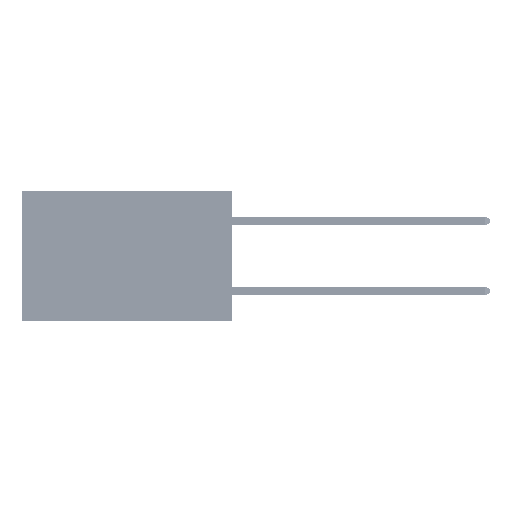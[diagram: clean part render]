
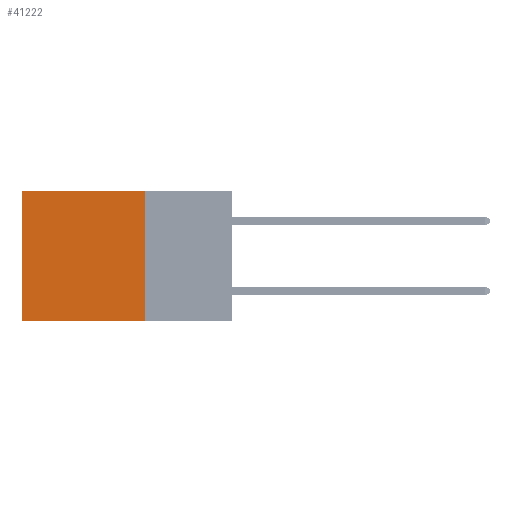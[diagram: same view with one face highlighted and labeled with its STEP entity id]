
A CAD part, left-side view. The second image highlights one B-rep face of the part: STEP entity #41222.
In plain terms, the highlighted planar face has unit normal (-1, 0, 0).
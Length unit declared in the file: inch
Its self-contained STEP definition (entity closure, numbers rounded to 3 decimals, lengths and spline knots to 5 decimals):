
#3738 = DIRECTION ( 'NONE',  ( 0., 1., 0. ) ) ;
#4277 = AXIS2_PLACEMENT_3D ( 'NONE', #21222, #21552, #17971 ) ;
#8140 = VERTEX_POINT ( 'NONE', #16720 ) ;
#9993 = ORIENTED_EDGE ( 'NONE', *, *, #18196, .F. ) ;
#10062 = ORIENTED_EDGE ( 'NONE', *, *, #41769, .T. ) ;
#10303 = LINE ( 'NONE', #29933, #22458 ) ;
#11612 = CARTESIAN_POINT ( 'NONE',  ( 0.2875, 0.6, -0.37 ) ) ;
#13410 = CARTESIAN_POINT ( 'NONE',  ( 0.2875, 0.25, 0. ) ) ;
#13441 = VECTOR ( 'NONE', #30210, 39.37008 ) ;
#13952 = FACE_OUTER_BOUND ( 'NONE', #19713, .T. ) ;
#15434 = VERTEX_POINT ( 'NONE', #11612 ) ;
#15583 = EDGE_CURVE ( 'NONE', #8140, #15434, #29682, .T. ) ;
#16121 = VERTEX_POINT ( 'NONE', #13410 ) ;
#16720 = CARTESIAN_POINT ( 'NONE',  ( 0.2875, 0.25, -0.37 ) ) ;
#17971 = DIRECTION ( 'NONE',  ( 0., 0., -1. ) ) ;
#18196 = EDGE_CURVE ( 'NONE', #16121, #8140, #10303, .T. ) ;
#18726 = ORIENTED_EDGE ( 'NONE', *, *, #15583, .F. ) ;
#19713 = EDGE_LOOP ( 'NONE', ( #10062, #18726, #9993, #26132 ) ) ;
#21222 = CARTESIAN_POINT ( 'NONE',  ( 0.2875, 0.25, 0. ) ) ;
#21552 = DIRECTION ( 'NONE',  ( 1., 0., 0. ) ) ;
#22458 = VECTOR ( 'NONE', #45708, 39.37008 ) ;
#23708 = VECTOR ( 'NONE', #25087, 39.37008 ) ;
#25087 = DIRECTION ( 'NONE',  ( 0., 0., -1. ) ) ;
#26086 = CARTESIAN_POINT ( 'NONE',  ( 0.2875, 0.25, -0.37 ) ) ;
#26132 = ORIENTED_EDGE ( 'NONE', *, *, #40349, .T. ) ;
#26750 = CARTESIAN_POINT ( 'NONE',  ( 0.2875, 0.6, 0. ) ) ;
#28347 = LINE ( 'NONE', #47556, #23708 ) ;
#28496 = LINE ( 'NONE', #33422, #13441 ) ;
#29682 = LINE ( 'NONE', #26086, #47004 ) ;
#29933 = CARTESIAN_POINT ( 'NONE',  ( 0.2875, 0.25, 0. ) ) ;
#30210 = DIRECTION ( 'NONE',  ( 0., 1., 0. ) ) ;
#33422 = CARTESIAN_POINT ( 'NONE',  ( 0.2875, 0.25, 0. ) ) ;
#40110 = PLANE ( 'NONE',  #4277 ) ;
#40349 = EDGE_CURVE ( 'NONE', #16121, #46318, #28496, .T. ) ;
#41222 = ADVANCED_FACE ( 'NONE', ( #13952 ), #40110, .F. ) ;
#41769 = EDGE_CURVE ( 'NONE', #46318, #15434, #28347, .T. ) ;
#45708 = DIRECTION ( 'NONE',  ( 0., 0., -1. ) ) ;
#46318 = VERTEX_POINT ( 'NONE', #26750 ) ;
#47004 = VECTOR ( 'NONE', #3738, 39.37008 ) ;
#47556 = CARTESIAN_POINT ( 'NONE',  ( 0.2875, 0.6, 0. ) ) ;
